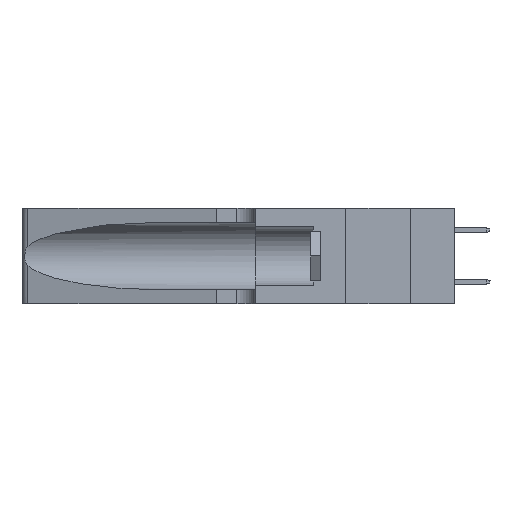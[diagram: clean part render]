
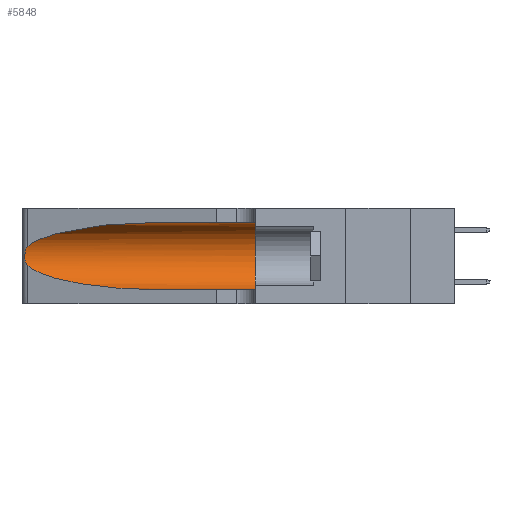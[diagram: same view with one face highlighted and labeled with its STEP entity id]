
A CAD part, left-side view. The second image highlights one B-rep face of the part: STEP entity #5848.
In plain terms, the highlighted cylindrical face has radius 3.308 mm (diameter 6.617 mm), a partial arc.
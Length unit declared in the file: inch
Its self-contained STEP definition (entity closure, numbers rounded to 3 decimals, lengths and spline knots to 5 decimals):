
#2693 = CARTESIAN_POINT ( 'NONE',  ( 0.25555, 1.22993, 0.14849 ) ) ;
#2743 = ORIENTED_EDGE ( 'NONE', *, *, #18050, .T. ) ;
#2917 = AXIS2_PLACEMENT_3D ( 'NONE', #32426, #5211, #32613 ) ;
#3754 = CARTESIAN_POINT ( 'NONE',  ( 0.18966, 0.96281, 0.31525 ) ) ;
#3915 = CIRCLE ( 'NONE', #28003, 0.13025 ) ;
#5072 = DIRECTION ( 'NONE',  ( 0., 0., 1. ) ) ;
#5211 = DIRECTION ( 'NONE',  ( 0., -1., 0. ) ) ;
#5512 = CARTESIAN_POINT ( 'NONE',  ( 0.1305, 1.61858, 0.05475 ) ) ;
#5656 = CARTESIAN_POINT ( 'NONE',  ( 0.26075, 1.23896, 0.178 ) ) ;
#5848 = ADVANCED_FACE ( 'NONE', ( #23231 ), #11353, .F. ) ;
#5849 = CARTESIAN_POINT ( 'NONE',  ( 0.26017, 1.23833, 0.17102 ) ) ;
#6404 = VERTEX_POINT ( 'NONE', #28146 ) ;
#6438 = CARTESIAN_POINT ( 'NONE',  ( 0.25487, 1.22718, 0.22369 ) ) ;
#7691 = LINE ( 'NONE', #5512, #11588 ) ;
#8809 = CARTESIAN_POINT ( 'NONE',  ( 0.26075, 1.23896, 0.19203 ) ) ;
#8935 = VERTEX_POINT ( 'NONE', #20074 ) ;
#9746 = VERTEX_POINT ( 'NONE', #36367 ) ;
#9840 = EDGE_CURVE ( 'NONE', #6404, #27559, #16832, .T. ) ;
#10378 = VERTEX_POINT ( 'NONE', #29363 ) ;
#11353 = CYLINDRICAL_SURFACE ( 'NONE', #2917, 0.13025 ) ;
#11588 = VECTOR ( 'NONE', #29922, 39.37008 ) ;
#11609 = CARTESIAN_POINT ( 'NONE',  ( 0.25854, 1.2359, 0.20912 ) ) ;
#11885 = CARTESIAN_POINT ( 'NONE',  ( 0.18966, 0.96281, 0.05475 ) ) ;
#11984 = CARTESIAN_POINT ( 'NONE',  ( 0.25787, 1.23484, 0.2124 ) ) ;
#13653 = CARTESIAN_POINT ( 'NONE',  ( 0.2373, 1.15595, 0.28018 ) ) ;
#14176 = ORIENTED_EDGE ( 'NONE', *, *, #18450, .F. ) ;
#14323 = B_SPLINE_CURVE_WITH_KNOTS ( 'NONE', 3,
 ( #17543, #29673, #38862, #11984, #11609, #23686, #8809, #5656, #5849, #30057, #21066, #17729, #2693, #14770 ),
 .UNSPECIFIED., .F., .F.,
 ( 4, 2, 2, 2, 2, 2, 4 ),
 ( 0., 0.00027, 0.00053, 0.00107, 0.0016, 0.00187, 0.00214 ),
 .UNSPECIFIED. ) ;
#14770 = CARTESIAN_POINT ( 'NONE',  ( 0.25487, 1.22718, 0.14631 ) ) ;
#15302 = ORIENTED_EDGE ( 'NONE', *, *, #29107, .T. ) ;
#15774 = ORIENTED_EDGE ( 'NONE', *, *, #23863, .T. ) ;
#16239 = CARTESIAN_POINT ( 'NONE',  ( 0.1305, 0.72297, 0.31525 ) ) ;
#16832 = LINE ( 'NONE', #19404, #28348 ) ;
#17543 = CARTESIAN_POINT ( 'NONE',  ( 0.25487, 1.22718, 0.22369 ) ) ;
#17729 = CARTESIAN_POINT ( 'NONE',  ( 0.25639, 1.23186, 0.15144 ) ) ;
#18050 = EDGE_CURVE ( 'NONE', #33740, #10378, #14323, .T. ) ;
#18450 = EDGE_CURVE ( 'NONE', #27559, #9746, #3915, .T. ) ;
#19404 = CARTESIAN_POINT ( 'NONE',  ( 0.1305, 1.61858, 0.31525 ) ) ;
#19845 =( BOUNDED_CURVE ( )  B_SPLINE_CURVE ( 3, ( #16239, #3754, #13653, #28349 ),
 .UNSPECIFIED., .F., .F. ) 
 B_SPLINE_CURVE_WITH_KNOTS ( ( 4, 4 ),
 ( 1.5708, 2.84003 ),
 .UNSPECIFIED. ) 
 CURVE ( )  GEOMETRIC_REPRESENTATION_ITEM ( )  RATIONAL_B_SPLINE_CURVE ( ( 1., 0.87, 0.87, 1. ) ) 
 REPRESENTATION_ITEM ( '' )  );
#20074 = CARTESIAN_POINT ( 'NONE',  ( 0.1305, 0.72297, 0.05475 ) ) ;
#21066 = CARTESIAN_POINT ( 'NONE',  ( 0.25789, 1.23486, 0.15765 ) ) ;
#22391 = EDGE_LOOP ( 'NONE', ( #15774, #2743, #23287, #15302, #14176, #27259 ) ) ;
#23231 = FACE_OUTER_BOUND ( 'NONE', #22391, .T. ) ;
#23287 = ORIENTED_EDGE ( 'NONE', *, *, #33836, .T. ) ;
#23686 = CARTESIAN_POINT ( 'NONE',  ( 0.26018, 1.23835, 0.19895 ) ) ;
#23863 = EDGE_CURVE ( 'NONE', #6404, #33740, #19845, .T. ) ;
#25739 = DIRECTION ( 'NONE',  ( 0., -1., 0. ) ) ;
#25817 = CARTESIAN_POINT ( 'NONE',  ( 0.2373, 1.15595, 0.08982 ) ) ;
#27259 = ORIENTED_EDGE ( 'NONE', *, *, #9840, .F. ) ;
#27559 = VERTEX_POINT ( 'NONE', #29733 ) ;
#28003 = AXIS2_PLACEMENT_3D ( 'NONE', #29491, #39065, #5072 ) ;
#28146 = CARTESIAN_POINT ( 'NONE',  ( 0.1305, 0.72297, 0.31525 ) ) ;
#28348 = VECTOR ( 'NONE', #25739, 39.37008 ) ;
#28349 = CARTESIAN_POINT ( 'NONE',  ( 0.25487, 1.22718, 0.22369 ) ) ;
#29107 = EDGE_CURVE ( 'NONE', #8935, #9746, #7691, .T. ) ;
#29363 = CARTESIAN_POINT ( 'NONE',  ( 0.25487, 1.22718, 0.14631 ) ) ;
#29491 = CARTESIAN_POINT ( 'NONE',  ( 0.1305, 0.35, 0.185 ) ) ;
#29673 = CARTESIAN_POINT ( 'NONE',  ( 0.25555, 1.22994, 0.2215 ) ) ;
#29733 = CARTESIAN_POINT ( 'NONE',  ( 0.1305, 0.35, 0.31525 ) ) ;
#29922 = DIRECTION ( 'NONE',  ( 0., -1., 0. ) ) ;
#30057 = CARTESIAN_POINT ( 'NONE',  ( 0.25856, 1.23593, 0.16098 ) ) ;
#32426 = CARTESIAN_POINT ( 'NONE',  ( 0.1305, 1.61858, 0.185 ) ) ;
#32613 = DIRECTION ( 'NONE',  ( 0., 0., -1. ) ) ;
#32764 = CARTESIAN_POINT ( 'NONE',  ( 0.25487, 1.22718, 0.14631 ) ) ;
#33740 = VERTEX_POINT ( 'NONE', #6438 ) ;
#33836 = EDGE_CURVE ( 'NONE', #10378, #8935, #36138, .T. ) ;
#36138 =( BOUNDED_CURVE ( )  B_SPLINE_CURVE ( 3, ( #32764, #25817, #11885, #38019 ),
 .UNSPECIFIED., .F., .T. ) 
 B_SPLINE_CURVE_WITH_KNOTS ( ( 4, 4 ),
 ( 3.44316, 4.71239 ),
 .UNSPECIFIED. ) 
 CURVE ( )  GEOMETRIC_REPRESENTATION_ITEM ( )  RATIONAL_B_SPLINE_CURVE ( ( 1., 0.87, 0.87, 1. ) ) 
 REPRESENTATION_ITEM ( '' )  );
#36367 = CARTESIAN_POINT ( 'NONE',  ( 0.1305, 0.35, 0.05475 ) ) ;
#38019 = CARTESIAN_POINT ( 'NONE',  ( 0.1305, 0.72297, 0.05475 ) ) ;
#38862 = CARTESIAN_POINT ( 'NONE',  ( 0.25639, 1.23184, 0.21858 ) ) ;
#39065 = DIRECTION ( 'NONE',  ( 0., 1., 0. ) ) ;
